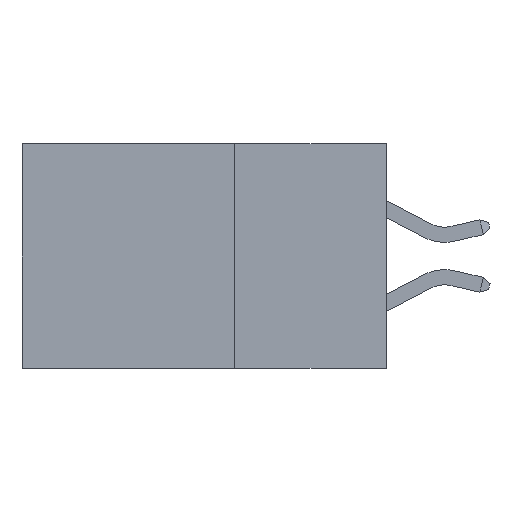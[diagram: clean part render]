
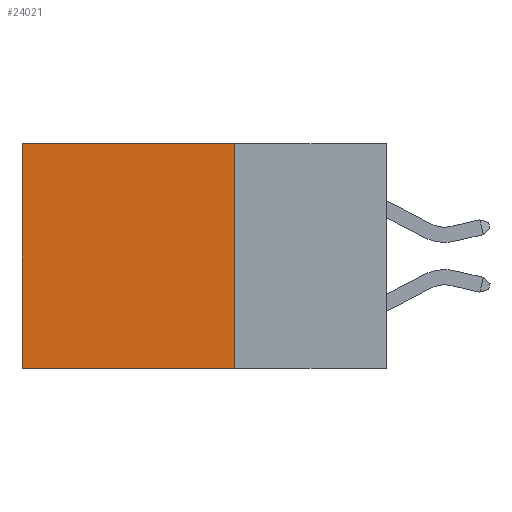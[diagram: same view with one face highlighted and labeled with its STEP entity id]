
A CAD part, left-side view. The second image highlights one B-rep face of the part: STEP entity #24021.
In plain terms, the highlighted planar face has unit normal (-1, 0, 0).
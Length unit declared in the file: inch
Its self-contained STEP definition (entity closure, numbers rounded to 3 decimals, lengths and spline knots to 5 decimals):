
#498 = DIRECTION ( 'NONE',  ( 0., 0., -1. ) ) ;
#3583 = EDGE_LOOP ( 'NONE', ( #4621, #6437, #12292, #12841 ) ) ;
#3695 = LINE ( 'NONE', #17909, #24124 ) ;
#3832 = CARTESIAN_POINT ( 'NONE',  ( 0.2615, 0.25, 0. ) ) ;
#4621 = ORIENTED_EDGE ( 'NONE', *, *, #12874, .T. ) ;
#5079 = CARTESIAN_POINT ( 'NONE',  ( 0.2615, 0.6, 0. ) ) ;
#6437 = ORIENTED_EDGE ( 'NONE', *, *, #18445, .F. ) ;
#6564 = CARTESIAN_POINT ( 'NONE',  ( 0.2615, 0.25, -0.37 ) ) ;
#8461 = VECTOR ( 'NONE', #14086, 39.37008 ) ;
#8985 = EDGE_CURVE ( 'NONE', #25709, #14928, #23978, .T. ) ;
#10712 = PLANE ( 'NONE',  #21661 ) ;
#11543 = CARTESIAN_POINT ( 'NONE',  ( 0.2615, 0.25, -0.37 ) ) ;
#12292 = ORIENTED_EDGE ( 'NONE', *, *, #19742, .F. ) ;
#12307 = CARTESIAN_POINT ( 'NONE',  ( 0.2615, 0.6, -0.37 ) ) ;
#12806 = DIRECTION ( 'NONE',  ( 1., 0., 0. ) ) ;
#12841 = ORIENTED_EDGE ( 'NONE', *, *, #8985, .T. ) ;
#12874 = EDGE_CURVE ( 'NONE', #14928, #22772, #3695, .T. ) ;
#13179 = VECTOR ( 'NONE', #20424, 39.37008 ) ;
#14086 = DIRECTION ( 'NONE',  ( 0., 1., 0. ) ) ;
#14602 = LINE ( 'NONE', #24187, #8461 ) ;
#14928 = VERTEX_POINT ( 'NONE', #5079 ) ;
#16187 = FACE_OUTER_BOUND ( 'NONE', #3583, .T. ) ;
#16337 = CARTESIAN_POINT ( 'NONE',  ( 0.2615, 0.25, -0.37 ) ) ;
#17909 = CARTESIAN_POINT ( 'NONE',  ( 0.2615, 0.6, -0.37 ) ) ;
#18445 = EDGE_CURVE ( 'NONE', #25549, #22772, #14602, .T. ) ;
#19742 = EDGE_CURVE ( 'NONE', #25709, #25549, #21218, .T. ) ;
#19960 = DIRECTION ( 'NONE',  ( 0., 0., -1. ) ) ;
#20424 = DIRECTION ( 'NONE',  ( 0., 1., 0. ) ) ;
#20537 = CARTESIAN_POINT ( 'NONE',  ( 0.2615, 0.25, 0. ) ) ;
#21218 = LINE ( 'NONE', #16337, #25930 ) ;
#21661 = AXIS2_PLACEMENT_3D ( 'NONE', #6564, #12806, #498 ) ;
#22463 = DIRECTION ( 'NONE',  ( 0., 0., -1. ) ) ;
#22772 = VERTEX_POINT ( 'NONE', #12307 ) ;
#23978 = LINE ( 'NONE', #20537, #13179 ) ;
#24021 = ADVANCED_FACE ( 'NONE', ( #16187 ), #10712, .F. ) ;
#24124 = VECTOR ( 'NONE', #19960, 39.37008 ) ;
#24187 = CARTESIAN_POINT ( 'NONE',  ( 0.2615, 0.25, -0.37 ) ) ;
#25549 = VERTEX_POINT ( 'NONE', #11543 ) ;
#25709 = VERTEX_POINT ( 'NONE', #3832 ) ;
#25930 = VECTOR ( 'NONE', #22463, 39.37008 ) ;
